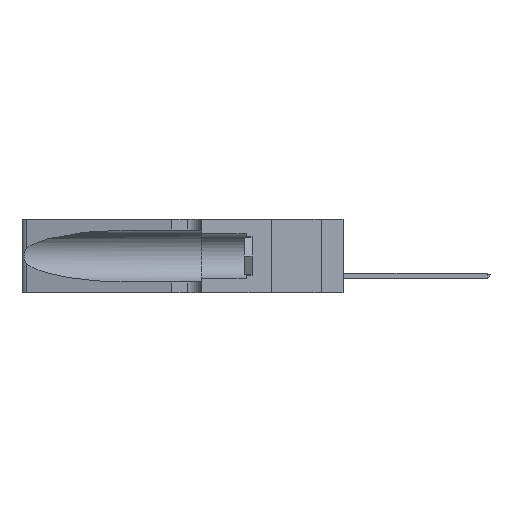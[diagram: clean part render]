
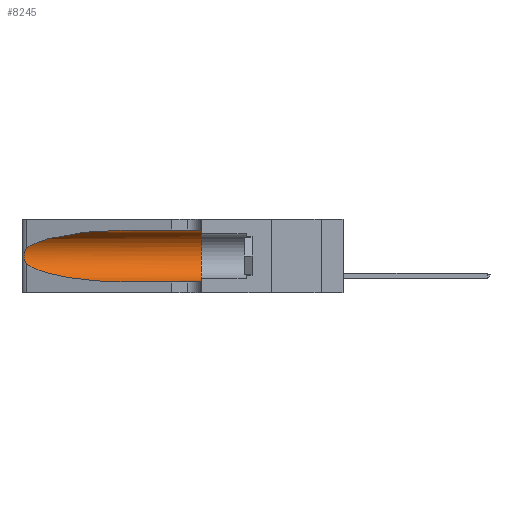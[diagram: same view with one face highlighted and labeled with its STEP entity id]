
A CAD part, left-side view. The second image highlights one B-rep face of the part: STEP entity #8245.
In plain terms, the highlighted cylindrical face has radius 3.308 mm (diameter 6.617 mm), a partial arc.
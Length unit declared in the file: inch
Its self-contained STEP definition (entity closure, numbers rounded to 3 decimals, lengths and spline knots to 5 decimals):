
#5 = CARTESIAN_POINT ( 'NONE',  ( 0.25555, 1.22994, 0.2215 ) ) ;
#305 = CARTESIAN_POINT ( 'NONE',  ( 0.1305, 0.72297, 0.05475 ) ) ;
#575 = ORIENTED_EDGE ( 'NONE', *, *, #26314, .F. ) ;
#714 = DIRECTION ( 'NONE',  ( 0., -1., 0. ) ) ;
#1565 = VECTOR ( 'NONE', #21531, 39.37008 ) ;
#1916 = CARTESIAN_POINT ( 'NONE',  ( 0.26018, 1.23835, 0.19895 ) ) ;
#2110 = FACE_OUTER_BOUND ( 'NONE', #17284, .T. ) ;
#2136 = CARTESIAN_POINT ( 'NONE',  ( 0.1305, 1.61858, 0.31525 ) ) ;
#2373 = CARTESIAN_POINT ( 'NONE',  ( 0.26017, 1.23833, 0.17102 ) ) ;
#3671 = VERTEX_POINT ( 'NONE', #6134 ) ;
#4560 =( BOUNDED_CURVE ( )  B_SPLINE_CURVE ( 3, ( #20407, #7333, #20305, #22566 ),
 .UNSPECIFIED., .F., .F. ) 
 B_SPLINE_CURVE_WITH_KNOTS ( ( 4, 4 ),
 ( 3.44316, 4.71239 ),
 .UNSPECIFIED. ) 
 CURVE ( )  GEOMETRIC_REPRESENTATION_ITEM ( )  RATIONAL_B_SPLINE_CURVE ( ( 1., 0.87, 0.87, 1. ) ) 
 REPRESENTATION_ITEM ( '' )  );
#4838 = ORIENTED_EDGE ( 'NONE', *, *, #13887, .T. ) ;
#4996 = CARTESIAN_POINT ( 'NONE',  ( 0.1305, 0.35, 0.185 ) ) ;
#6134 = CARTESIAN_POINT ( 'NONE',  ( 0.1305, 0.72297, 0.31525 ) ) ;
#6171 = CARTESIAN_POINT ( 'NONE',  ( 0.25487, 1.22718, 0.22369 ) ) ;
#6199 = CARTESIAN_POINT ( 'NONE',  ( 0.25487, 1.22718, 0.14631 ) ) ;
#6251 = CARTESIAN_POINT ( 'NONE',  ( 0.26075, 1.23896, 0.178 ) ) ;
#6302 = VERTEX_POINT ( 'NONE', #14079 ) ;
#6543 = CARTESIAN_POINT ( 'NONE',  ( 0.25854, 1.2359, 0.20912 ) ) ;
#6571 = DIRECTION ( 'NONE',  ( 0., 0., -1. ) ) ;
#6810 = CARTESIAN_POINT ( 'NONE',  ( 0.25555, 1.22993, 0.14849 ) ) ;
#6884 = CARTESIAN_POINT ( 'NONE',  ( 0.1305, 1.61858, 0.185 ) ) ;
#7109 = CIRCLE ( 'NONE', #25956, 0.13025 ) ;
#7299 = CARTESIAN_POINT ( 'NONE',  ( 0.25789, 1.23486, 0.15765 ) ) ;
#7333 = CARTESIAN_POINT ( 'NONE',  ( 0.2373, 1.15595, 0.08982 ) ) ;
#7534 = ORIENTED_EDGE ( 'NONE', *, *, #17357, .F. ) ;
#7935 = ORIENTED_EDGE ( 'NONE', *, *, #26880, .T. ) ;
#8245 = ADVANCED_FACE ( 'NONE', ( #2110 ), #19507, .F. ) ;
#8476 = CARTESIAN_POINT ( 'NONE',  ( 0.18966, 0.96281, 0.31525 ) ) ;
#8981 = EDGE_CURVE ( 'NONE', #19105, #19556, #15122, .T. ) ;
#10459 = CARTESIAN_POINT ( 'NONE',  ( 0.25487, 1.22718, 0.22369 ) ) ;
#12478 = CARTESIAN_POINT ( 'NONE',  ( 0.25487, 1.22718, 0.22369 ) ) ;
#12589 = ORIENTED_EDGE ( 'NONE', *, *, #14211, .T. ) ;
#12777 = CARTESIAN_POINT ( 'NONE',  ( 0.26075, 1.23896, 0.19203 ) ) ;
#13353 = DIRECTION ( 'NONE',  ( 0., -1., 0. ) ) ;
#13452 = AXIS2_PLACEMENT_3D ( 'NONE', #6884, #714, #6571 ) ;
#13887 = EDGE_CURVE ( 'NONE', #26240, #26689, #14540, .T. ) ;
#14079 = CARTESIAN_POINT ( 'NONE',  ( 0.1305, 0.35, 0.31525 ) ) ;
#14211 = EDGE_CURVE ( 'NONE', #19556, #26240, #4560, .T. ) ;
#14540 = LINE ( 'NONE', #16625, #1565 ) ;
#15122 = B_SPLINE_CURVE_WITH_KNOTS ( 'NONE', 3,
 ( #10459, #5, #25938, #15276, #6543, #1916, #12777, #6251, #2373, #20372, #7299, #24207, #6810, #26138 ),
 .UNSPECIFIED., .F., .F.,
 ( 4, 2, 2, 2, 2, 2, 4 ),
 ( 0., 0.00027, 0.00053, 0.00107, 0.0016, 0.00187, 0.00214 ),
 .UNSPECIFIED. ) ;
#15276 = CARTESIAN_POINT ( 'NONE',  ( 0.25787, 1.23484, 0.2124 ) ) ;
#16625 = CARTESIAN_POINT ( 'NONE',  ( 0.1305, 1.61858, 0.05475 ) ) ;
#17201 = ORIENTED_EDGE ( 'NONE', *, *, #8981, .T. ) ;
#17284 = EDGE_LOOP ( 'NONE', ( #7935, #17201, #12589, #4838, #7534, #575 ) ) ;
#17357 = EDGE_CURVE ( 'NONE', #6302, #26689, #7109, .T. ) ;
#19105 = VERTEX_POINT ( 'NONE', #12478 ) ;
#19507 = CYLINDRICAL_SURFACE ( 'NONE', #13452, 0.13025 ) ;
#19556 = VERTEX_POINT ( 'NONE', #6199 ) ;
#20278 = LINE ( 'NONE', #2136, #28069 ) ;
#20305 = CARTESIAN_POINT ( 'NONE',  ( 0.18966, 0.96281, 0.05475 ) ) ;
#20372 = CARTESIAN_POINT ( 'NONE',  ( 0.25856, 1.23593, 0.16098 ) ) ;
#20378 = DIRECTION ( 'NONE',  ( 0., 0., 1. ) ) ;
#20407 = CARTESIAN_POINT ( 'NONE',  ( 0.25487, 1.22718, 0.14631 ) ) ;
#21531 = DIRECTION ( 'NONE',  ( 0., -1., 0. ) ) ;
#21799 = CARTESIAN_POINT ( 'NONE',  ( 0.1305, 0.72297, 0.31525 ) ) ;
#22566 = CARTESIAN_POINT ( 'NONE',  ( 0.1305, 0.72297, 0.05475 ) ) ;
#23500 = CARTESIAN_POINT ( 'NONE',  ( 0.1305, 0.35, 0.05475 ) ) ;
#24207 = CARTESIAN_POINT ( 'NONE',  ( 0.25639, 1.23186, 0.15144 ) ) ;
#24796 =( BOUNDED_CURVE ( )  B_SPLINE_CURVE ( 3, ( #21799, #8476, #25943, #6171 ),
 .UNSPECIFIED., .F., .F. ) 
 B_SPLINE_CURVE_WITH_KNOTS ( ( 4, 4 ),
 ( 1.5708, 2.84003 ),
 .UNSPECIFIED. ) 
 CURVE ( )  GEOMETRIC_REPRESENTATION_ITEM ( )  RATIONAL_B_SPLINE_CURVE ( ( 1., 0.87, 0.87, 1. ) ) 
 REPRESENTATION_ITEM ( '' )  );
#25094 = DIRECTION ( 'NONE',  ( 0., 1., 0. ) ) ;
#25938 = CARTESIAN_POINT ( 'NONE',  ( 0.25639, 1.23184, 0.21858 ) ) ;
#25943 = CARTESIAN_POINT ( 'NONE',  ( 0.2373, 1.15595, 0.28018 ) ) ;
#25956 = AXIS2_PLACEMENT_3D ( 'NONE', #4996, #25094, #20378 ) ;
#26138 = CARTESIAN_POINT ( 'NONE',  ( 0.25487, 1.22718, 0.14631 ) ) ;
#26240 = VERTEX_POINT ( 'NONE', #305 ) ;
#26314 = EDGE_CURVE ( 'NONE', #3671, #6302, #20278, .T. ) ;
#26689 = VERTEX_POINT ( 'NONE', #23500 ) ;
#26880 = EDGE_CURVE ( 'NONE', #3671, #19105, #24796, .T. ) ;
#28069 = VECTOR ( 'NONE', #13353, 39.37008 ) ;
